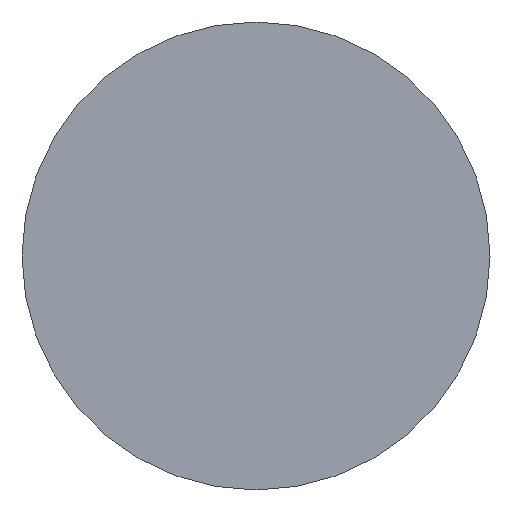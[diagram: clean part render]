
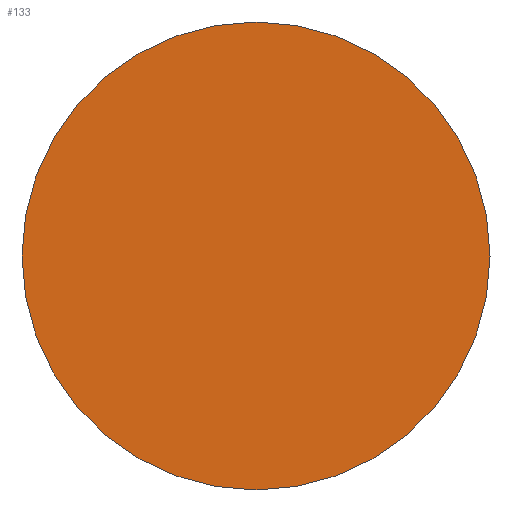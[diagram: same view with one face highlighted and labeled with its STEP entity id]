
A CAD part, left-side view. The second image highlights one B-rep face of the part: STEP entity #133.
In plain terms, the highlighted planar face has unit normal (-1, 0, 0).
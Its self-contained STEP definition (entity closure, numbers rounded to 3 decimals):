
#20 = DIRECTION ( 'NONE',  ( 0., 0., -1. ) ) ;
#21 = CARTESIAN_POINT ( 'NONE',  ( -19.41, 47.829, -20.721 ) ) ;
#26 = AXIS2_PLACEMENT_3D ( 'NONE', #21, #73, #124 ) ;
#31 = EDGE_CURVE ( 'NONE', #118, #159, #64, .T. ) ;
#42 = CARTESIAN_POINT ( 'NONE',  ( -19.41, 47.829, -20.721 ) ) ;
#55 = ORIENTED_EDGE ( 'NONE', *, *, #90, .F. ) ;
#58 = FACE_OUTER_BOUND ( 'NONE', #158, .T. ) ;
#64 = CIRCLE ( 'NONE', #104, 4. ) ;
#73 = DIRECTION ( 'NONE',  ( 1., 0., 0. ) ) ;
#78 = AXIS2_PLACEMENT_3D ( 'NONE', #137, #138, #20 ) ;
#79 = CIRCLE ( 'NONE', #78, 4. ) ;
#90 = EDGE_CURVE ( 'NONE', #159, #118, #79, .T. ) ;
#93 = DIRECTION ( 'NONE',  ( 0., 0., -1. ) ) ;
#104 = AXIS2_PLACEMENT_3D ( 'NONE', #42, #122, #93 ) ;
#109 = CARTESIAN_POINT ( 'NONE',  ( -19.41, 47.829, -24.721 ) ) ;
#110 = CARTESIAN_POINT ( 'NONE',  ( -19.41, 47.829, -16.721 ) ) ;
#118 = VERTEX_POINT ( 'NONE', #109 ) ;
#122 = DIRECTION ( 'NONE',  ( 1., 0., 0. ) ) ;
#124 = DIRECTION ( 'NONE',  ( 0., 0., -1. ) ) ;
#133 = ADVANCED_FACE ( '$', ( #58 ), #150, .F. ) ;
#137 = CARTESIAN_POINT ( 'NONE',  ( -19.41, 47.829, -20.721 ) ) ;
#138 = DIRECTION ( 'NONE',  ( 1., 0., 0. ) ) ;
#148 = ORIENTED_EDGE ( 'NONE', *, *, #31, .F. ) ;
#150 = PLANE ( 'NONE',  #26 ) ;
#158 = EDGE_LOOP ( 'NONE', ( #148, #55 ) ) ;
#159 = VERTEX_POINT ( 'NONE', #110 ) ;
